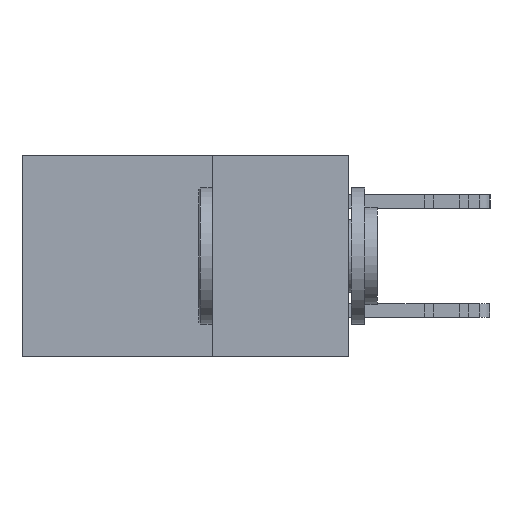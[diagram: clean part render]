
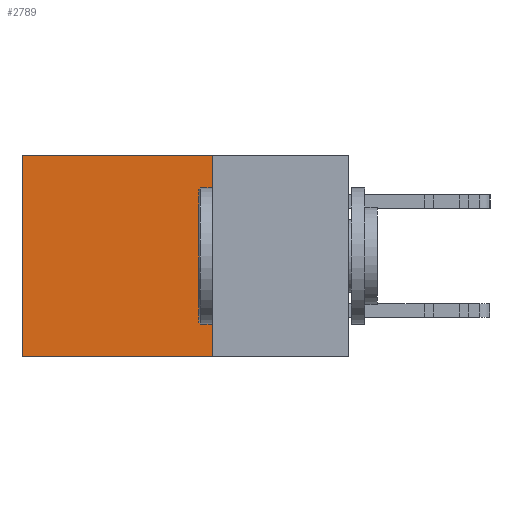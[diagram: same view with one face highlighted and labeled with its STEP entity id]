
A CAD part, left-side view. The second image highlights one B-rep face of the part: STEP entity #2789.
In plain terms, the highlighted planar face has unit normal (-1, 0, 0).
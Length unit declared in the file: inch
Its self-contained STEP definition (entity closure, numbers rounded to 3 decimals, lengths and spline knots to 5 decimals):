
#804 = ORIENTED_EDGE ( 'NONE', *, *, #11528, .F. ) ;
#1114 = EDGE_CURVE ( 'NONE', #19967, #5158, #20653, .T. ) ;
#2245 = LINE ( 'NONE', #19860, #10377 ) ;
#2789 = ADVANCED_FACE ( 'NONE', ( #20257 ), #14177, .F. ) ;
#3419 = VERTEX_POINT ( 'NONE', #22168 ) ;
#5158 = VERTEX_POINT ( 'NONE', #12420 ) ;
#6009 = CARTESIAN_POINT ( 'NONE',  ( 0.2615, 0.25, -0.37 ) ) ;
#6526 = ORIENTED_EDGE ( 'NONE', *, *, #15070, .T. ) ;
#6920 = VERTEX_POINT ( 'NONE', #12381 ) ;
#7153 = VECTOR ( 'NONE', #7508, 39.37008 ) ;
#7508 = DIRECTION ( 'NONE',  ( 0., 0., -1. ) ) ;
#7580 = ORIENTED_EDGE ( 'NONE', *, *, #18609, .F. ) ;
#9449 = LINE ( 'NONE', #13460, #7153 ) ;
#9770 = DIRECTION ( 'NONE',  ( 1., 0., 0. ) ) ;
#10377 = VECTOR ( 'NONE', #14416, 39.37008 ) ;
#11528 = EDGE_CURVE ( 'NONE', #19967, #3419, #9449, .T. ) ;
#11967 = DIRECTION ( 'NONE',  ( 0., 0., -1. ) ) ;
#12267 = VECTOR ( 'NONE', #23976, 39.37008 ) ;
#12381 = CARTESIAN_POINT ( 'NONE',  ( 0.2615, 0.6, -0.37 ) ) ;
#12420 = CARTESIAN_POINT ( 'NONE',  ( 0.2615, 0.6, 0. ) ) ;
#13460 = CARTESIAN_POINT ( 'NONE',  ( 0.2615, 0.25, -0.37 ) ) ;
#14177 = PLANE ( 'NONE',  #16007 ) ;
#14416 = DIRECTION ( 'NONE',  ( 0., 1., 0. ) ) ;
#14916 = EDGE_LOOP ( 'NONE', ( #6526, #7580, #804, #16788 ) ) ;
#15070 = EDGE_CURVE ( 'NONE', #5158, #6920, #18404, .T. ) ;
#16007 = AXIS2_PLACEMENT_3D ( 'NONE', #6009, #9770, #11967 ) ;
#16788 = ORIENTED_EDGE ( 'NONE', *, *, #1114, .T. ) ;
#18404 = LINE ( 'NONE', #24107, #12267 ) ;
#18609 = EDGE_CURVE ( 'NONE', #3419, #6920, #2245, .T. ) ;
#19860 = CARTESIAN_POINT ( 'NONE',  ( 0.2615, 0.25, -0.37 ) ) ;
#19967 = VERTEX_POINT ( 'NONE', #21801 ) ;
#20257 = FACE_OUTER_BOUND ( 'NONE', #14916, .T. ) ;
#20404 = CARTESIAN_POINT ( 'NONE',  ( 0.2615, 0.25, 0. ) ) ;
#20653 = LINE ( 'NONE', #20404, #23997 ) ;
#21801 = CARTESIAN_POINT ( 'NONE',  ( 0.2615, 0.25, 0. ) ) ;
#22168 = CARTESIAN_POINT ( 'NONE',  ( 0.2615, 0.25, -0.37 ) ) ;
#23976 = DIRECTION ( 'NONE',  ( 0., 0., -1. ) ) ;
#23997 = VECTOR ( 'NONE', #24541, 39.37008 ) ;
#24107 = CARTESIAN_POINT ( 'NONE',  ( 0.2615, 0.6, -0.37 ) ) ;
#24541 = DIRECTION ( 'NONE',  ( 0., 1., 0. ) ) ;
